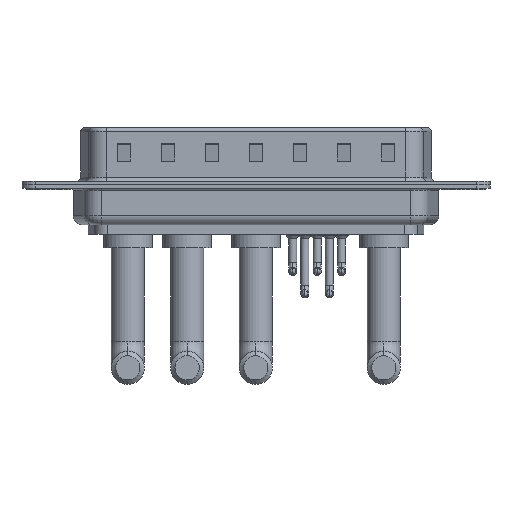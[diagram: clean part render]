
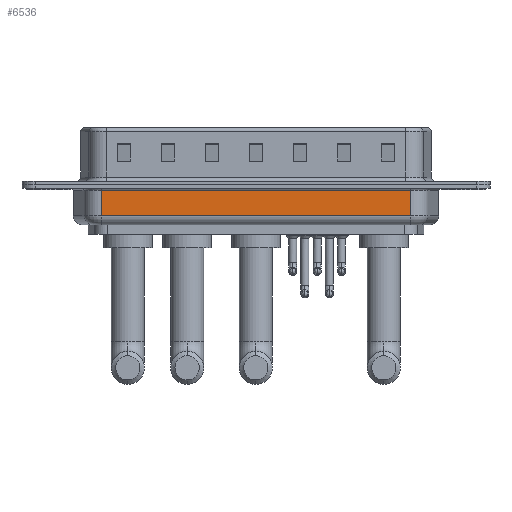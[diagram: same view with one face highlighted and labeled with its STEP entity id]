
A CAD part, front view. The second image highlights one B-rep face of the part: STEP entity #6536.
In plain terms, the highlighted planar face has unit normal (0, -1, 0).
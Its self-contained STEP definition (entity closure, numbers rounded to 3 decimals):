
#92 = DIRECTION ( 'NONE',  ( 1., 0., 0. ) ) ;
#783 = CARTESIAN_POINT ( 'NONE',  ( 6.006, -5.35, -3.5 ) ) ;
#1675 = CARTESIAN_POINT ( 'NONE',  ( 41.044, -5.35, -3.5 ) ) ;
#1805 = CARTESIAN_POINT ( 'NONE',  ( 6.006, -5.35, -4.5 ) ) ;
#2974 = ORIENTED_EDGE ( 'NONE', *, *, #6160, .F. ) ;
#3174 = VECTOR ( 'NONE', #5533, 1000. ) ;
#3433 = CARTESIAN_POINT ( 'NONE',  ( 41.044, -5.35, -0.65 ) ) ;
#3513 = VERTEX_POINT ( 'NONE', #3433 ) ;
#3582 = ORIENTED_EDGE ( 'NONE', *, *, #9530, .T. ) ;
#3805 = DIRECTION ( 'NONE',  ( 0., 0., 1. ) ) ;
#4521 = EDGE_CURVE ( 'NONE', #7043, #3513, #15678, .T. ) ;
#4873 = LINE ( 'NONE', #17638, #5865 ) ;
#5043 = LINE ( 'NONE', #13592, #3174 ) ;
#5533 = DIRECTION ( 'NONE',  ( -1., 0., 0. ) ) ;
#5748 = EDGE_LOOP ( 'NONE', ( #2974, #17629, #18193, #3582 ) ) ;
#5865 = VECTOR ( 'NONE', #92, 1000. ) ;
#6160 = EDGE_CURVE ( 'NONE', #20659, #7107, #10013, .T. ) ;
#6536 = ADVANCED_FACE ( 'NONE', ( #17481 ), #17800, .F. ) ;
#7043 = VERTEX_POINT ( 'NONE', #1675 ) ;
#7065 = VECTOR ( 'NONE', #14116, 1000. ) ;
#7107 = VERTEX_POINT ( 'NONE', #19442 ) ;
#9422 = AXIS2_PLACEMENT_3D ( 'NONE', #1805, #12997, #14665 ) ;
#9530 = EDGE_CURVE ( 'NONE', #3513, #7107, #5043, .T. ) ;
#10013 = LINE ( 'NONE', #11972, #17423 ) ;
#10990 = CARTESIAN_POINT ( 'NONE',  ( 41.044, -5.35, -4.5 ) ) ;
#11972 = CARTESIAN_POINT ( 'NONE',  ( 6.006, -5.35, -4.5 ) ) ;
#12997 = DIRECTION ( 'NONE',  ( 0., 1., 0. ) ) ;
#13592 = CARTESIAN_POINT ( 'NONE',  ( 6.006, -5.35, -0.65 ) ) ;
#14116 = DIRECTION ( 'NONE',  ( 0., 0., 1. ) ) ;
#14665 = DIRECTION ( 'NONE',  ( 0., 0., 1. ) ) ;
#15477 = EDGE_CURVE ( 'NONE', #20659, #7043, #4873, .T. ) ;
#15678 = LINE ( 'NONE', #10990, #7065 ) ;
#17423 = VECTOR ( 'NONE', #3805, 1000. ) ;
#17481 = FACE_OUTER_BOUND ( 'NONE', #5748, .T. ) ;
#17629 = ORIENTED_EDGE ( 'NONE', *, *, #15477, .T. ) ;
#17638 = CARTESIAN_POINT ( 'NONE',  ( 6.006, -5.35, -3.5 ) ) ;
#17800 = PLANE ( 'NONE',  #9422 ) ;
#18193 = ORIENTED_EDGE ( 'NONE', *, *, #4521, .T. ) ;
#19442 = CARTESIAN_POINT ( 'NONE',  ( 6.006, -5.35, -0.65 ) ) ;
#20659 = VERTEX_POINT ( 'NONE', #783 ) ;
